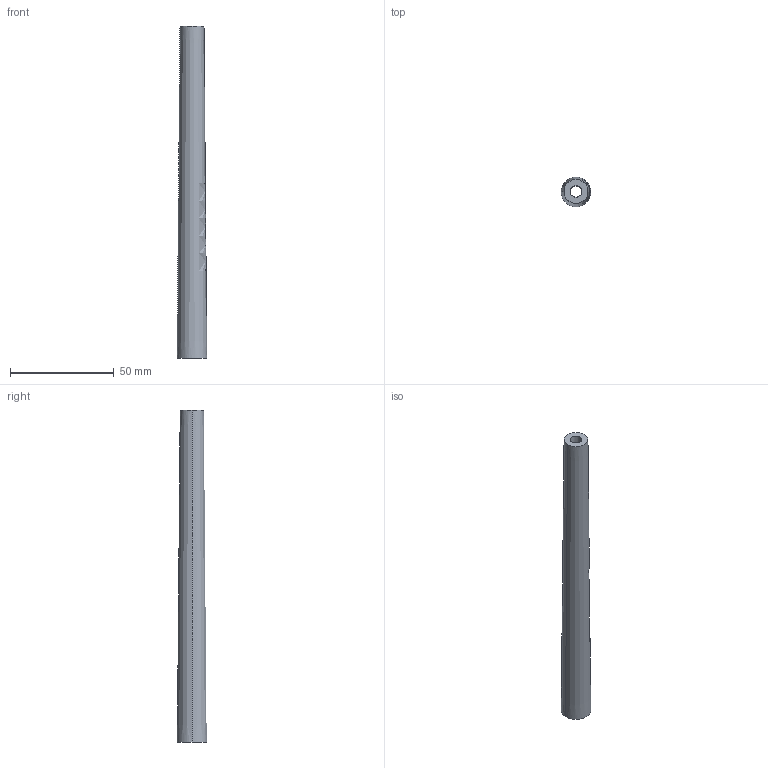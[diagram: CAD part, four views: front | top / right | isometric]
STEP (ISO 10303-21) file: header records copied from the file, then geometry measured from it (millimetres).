
FILE_DESCRIPTION (( 'STEP AP214' ), '1' );
FILE_NAME ('Barrel^StikM1.STEP', '2013-09-01T22:39:20', ( 'Asher' ), ( '' ), 'SwSTEP 2.0', 'SolidWorks 2013', '' );
FILE_SCHEMA (( 'AUTOMOTIVE_DESIGN' ));
Length unit declared in the file: millimetre
Products named in the file (1): Barrel^StikM1
Bounding box: 14.35 x 14.35 x 160 mm (x, y, z)
Volume: 17224.5 mm3; surface area: 9657 mm2
Topology: 1 solids, 1 shells, 367 faces, 1068 edges, 712 vertices
Faces by surface type: bspline 198, plane 149, cone 18, cylinder 2
Entity records: 19733 total; most frequent: CARTESIAN_POINT 11519, ORIENTED_EDGE 2136, EDGE_CURVE 1068, DIRECTION 987, VERTEX_POINT 712, LINE 487, VECTOR 487, B_SPLINE_CURVE_WITH_KNOTS 479
